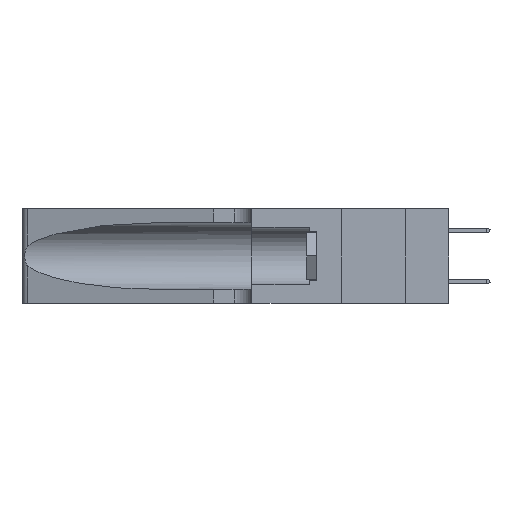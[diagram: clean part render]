
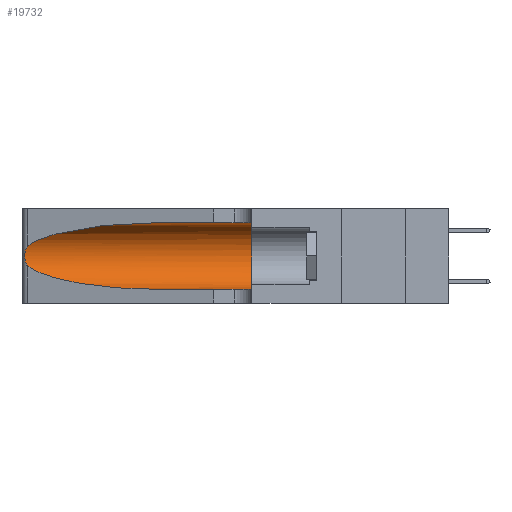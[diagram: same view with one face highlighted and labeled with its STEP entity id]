
A CAD part, left-side view. The second image highlights one B-rep face of the part: STEP entity #19732.
In plain terms, the highlighted cylindrical face has radius 3.308 mm (diameter 6.617 mm), a partial arc.
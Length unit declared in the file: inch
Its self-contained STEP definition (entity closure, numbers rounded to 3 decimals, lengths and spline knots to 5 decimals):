
#59 = ORIENTED_EDGE ( 'NONE', *, *, #25251, .F. ) ;
#1395 = VERTEX_POINT ( 'NONE', #16556 ) ;
#1574 = CARTESIAN_POINT ( 'NONE',  ( 0.1305, 1.61858, 0.05475 ) ) ;
#2833 = VERTEX_POINT ( 'NONE', #46122 ) ;
#2888 = VECTOR ( 'NONE', #8637, 39.37008 ) ;
#4308 = FACE_OUTER_BOUND ( 'NONE', #15953, .T. ) ;
#4635 = ORIENTED_EDGE ( 'NONE', *, *, #43085, .T. ) ;
#5262 = DIRECTION ( 'NONE',  ( 0., -1., 0. ) ) ;
#6433 = CARTESIAN_POINT ( 'NONE',  ( 0.25787, 1.23484, 0.2124 ) ) ;
#7779 =( BOUNDED_CURVE ( )  B_SPLINE_CURVE ( 3, ( #31865, #38965, #21337, #46109 ),
 .UNSPECIFIED., .F., .F. ) 
 B_SPLINE_CURVE_WITH_KNOTS ( ( 4, 4 ),
 ( 1.5708, 2.84003 ),
 .UNSPECIFIED. ) 
 CURVE ( )  GEOMETRIC_REPRESENTATION_ITEM ( )  RATIONAL_B_SPLINE_CURVE ( ( 1., 0.87, 0.87, 1. ) ) 
 REPRESENTATION_ITEM ( '' )  );
#8637 = DIRECTION ( 'NONE',  ( 0., -1., 0. ) ) ;
#9942 = EDGE_CURVE ( 'NONE', #2833, #10032, #11317, .T. ) ;
#10032 = VERTEX_POINT ( 'NONE', #17921 ) ;
#10181 = CARTESIAN_POINT ( 'NONE',  ( 0.26018, 1.23835, 0.19895 ) ) ;
#11317 = B_SPLINE_CURVE_WITH_KNOTS ( 'NONE', 3,
 ( #20835, #13533, #27980, #6433, #31501, #10181, #35091, #13822, #38610, #17454, #42158, #20970, #45749, #24536 ),
 .UNSPECIFIED., .F., .F.,
 ( 4, 2, 2, 2, 2, 2, 4 ),
 ( 0., 0.00027, 0.00053, 0.00107, 0.0016, 0.00187, 0.00214 ),
 .UNSPECIFIED. ) ;
#11552 = AXIS2_PLACEMENT_3D ( 'NONE', #40693, #40549, #19519 ) ;
#11901 = DIRECTION ( 'NONE',  ( 0., 1., 0. ) ) ;
#12268 = CARTESIAN_POINT ( 'NONE',  ( 0.1305, 0.72297, 0.05475 ) ) ;
#13533 = CARTESIAN_POINT ( 'NONE',  ( 0.25555, 1.22994, 0.2215 ) ) ;
#13822 = CARTESIAN_POINT ( 'NONE',  ( 0.26075, 1.23896, 0.178 ) ) ;
#13883 = CARTESIAN_POINT ( 'NONE',  ( 0.1305, 0.72297, 0.31525 ) ) ;
#15756 = CARTESIAN_POINT ( 'NONE',  ( 0.25487, 1.22718, 0.14631 ) ) ;
#15953 = EDGE_LOOP ( 'NONE', ( #45421, #18310, #4635, #24403, #34956, #59 ) ) ;
#16556 = CARTESIAN_POINT ( 'NONE',  ( 0.1305, 0.72297, 0.05475 ) ) ;
#17454 = CARTESIAN_POINT ( 'NONE',  ( 0.25856, 1.23593, 0.16098 ) ) ;
#17921 = CARTESIAN_POINT ( 'NONE',  ( 0.25487, 1.22718, 0.14631 ) ) ;
#18254 = VECTOR ( 'NONE', #5262, 39.37008 ) ;
#18310 = ORIENTED_EDGE ( 'NONE', *, *, #9942, .T. ) ;
#19519 = DIRECTION ( 'NONE',  ( 0., 0., -1. ) ) ;
#19577 = VERTEX_POINT ( 'NONE', #25860 ) ;
#19732 = ADVANCED_FACE ( 'NONE', ( #4308 ), #31808, .F. ) ;
#20835 = CARTESIAN_POINT ( 'NONE',  ( 0.25487, 1.22718, 0.22369 ) ) ;
#20970 = CARTESIAN_POINT ( 'NONE',  ( 0.25639, 1.23186, 0.15144 ) ) ;
#21337 = CARTESIAN_POINT ( 'NONE',  ( 0.2373, 1.15595, 0.28018 ) ) ;
#22889 = CARTESIAN_POINT ( 'NONE',  ( 0.2373, 1.15595, 0.08982 ) ) ;
#24403 = ORIENTED_EDGE ( 'NONE', *, *, #26722, .T. ) ;
#24536 = CARTESIAN_POINT ( 'NONE',  ( 0.25487, 1.22718, 0.14631 ) ) ;
#25251 = EDGE_CURVE ( 'NONE', #31202, #44848, #31577, .T. ) ;
#25860 = CARTESIAN_POINT ( 'NONE',  ( 0.1305, 0.35, 0.05475 ) ) ;
#26722 = EDGE_CURVE ( 'NONE', #1395, #19577, #37071, .T. ) ;
#27980 = CARTESIAN_POINT ( 'NONE',  ( 0.25639, 1.23184, 0.21858 ) ) ;
#29301 =( BOUNDED_CURVE ( )  B_SPLINE_CURVE ( 3, ( #15756, #22889, #33543, #12268 ),
 .UNSPECIFIED., .F., .F. ) 
 B_SPLINE_CURVE_WITH_KNOTS ( ( 4, 4 ),
 ( 3.44316, 4.71239 ),
 .UNSPECIFIED. ) 
 CURVE ( )  GEOMETRIC_REPRESENTATION_ITEM ( )  RATIONAL_B_SPLINE_CURVE ( ( 1., 0.87, 0.87, 1. ) ) 
 REPRESENTATION_ITEM ( '' )  );
#29875 = CARTESIAN_POINT ( 'NONE',  ( 0.1305, 1.61858, 0.31525 ) ) ;
#30178 = CARTESIAN_POINT ( 'NONE',  ( 0.1305, 0.35, 0.31525 ) ) ;
#31202 = VERTEX_POINT ( 'NONE', #13883 ) ;
#31265 = EDGE_CURVE ( 'NONE', #31202, #2833, #7779, .T. ) ;
#31501 = CARTESIAN_POINT ( 'NONE',  ( 0.25854, 1.2359, 0.20912 ) ) ;
#31577 = LINE ( 'NONE', #29875, #2888 ) ;
#31808 = CYLINDRICAL_SURFACE ( 'NONE', #11552, 0.13025 ) ;
#31865 = CARTESIAN_POINT ( 'NONE',  ( 0.1305, 0.72297, 0.31525 ) ) ;
#33190 = CARTESIAN_POINT ( 'NONE',  ( 0.1305, 0.35, 0.185 ) ) ;
#33543 = CARTESIAN_POINT ( 'NONE',  ( 0.18966, 0.96281, 0.05475 ) ) ;
#33810 = CIRCLE ( 'NONE', #34252, 0.13025 ) ;
#34252 = AXIS2_PLACEMENT_3D ( 'NONE', #33190, #11901, #36763 ) ;
#34956 = ORIENTED_EDGE ( 'NONE', *, *, #41669, .F. ) ;
#35091 = CARTESIAN_POINT ( 'NONE',  ( 0.26075, 1.23896, 0.19203 ) ) ;
#36763 = DIRECTION ( 'NONE',  ( 0., 0., 1. ) ) ;
#37071 = LINE ( 'NONE', #1574, #18254 ) ;
#38610 = CARTESIAN_POINT ( 'NONE',  ( 0.26017, 1.23833, 0.17102 ) ) ;
#38965 = CARTESIAN_POINT ( 'NONE',  ( 0.18966, 0.96281, 0.31525 ) ) ;
#40549 = DIRECTION ( 'NONE',  ( 0., -1., 0. ) ) ;
#40693 = CARTESIAN_POINT ( 'NONE',  ( 0.1305, 1.61858, 0.185 ) ) ;
#41669 = EDGE_CURVE ( 'NONE', #44848, #19577, #33810, .T. ) ;
#42158 = CARTESIAN_POINT ( 'NONE',  ( 0.25789, 1.23486, 0.15765 ) ) ;
#43085 = EDGE_CURVE ( 'NONE', #10032, #1395, #29301, .T. ) ;
#44848 = VERTEX_POINT ( 'NONE', #30178 ) ;
#45421 = ORIENTED_EDGE ( 'NONE', *, *, #31265, .T. ) ;
#45749 = CARTESIAN_POINT ( 'NONE',  ( 0.25555, 1.22993, 0.14849 ) ) ;
#46109 = CARTESIAN_POINT ( 'NONE',  ( 0.25487, 1.22718, 0.22369 ) ) ;
#46122 = CARTESIAN_POINT ( 'NONE',  ( 0.25487, 1.22718, 0.22369 ) ) ;
